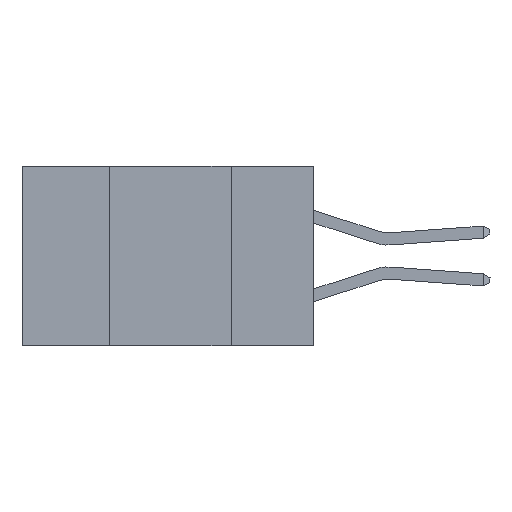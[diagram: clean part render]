
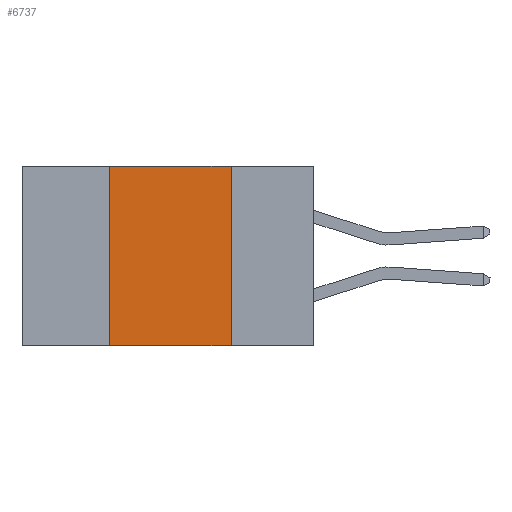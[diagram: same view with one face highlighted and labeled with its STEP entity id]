
A CAD part, left-side view. The second image highlights one B-rep face of the part: STEP entity #6737.
In plain terms, the highlighted planar face has unit normal (-1, 0, 0).
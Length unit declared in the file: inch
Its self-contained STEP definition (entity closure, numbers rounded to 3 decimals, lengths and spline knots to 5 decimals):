
#291 = EDGE_CURVE ( 'NONE', #8568, #8431, #4591, .T. ) ;
#351 = CARTESIAN_POINT ( 'NONE',  ( 0., 0.17, 0. ) ) ;
#398 = CARTESIAN_POINT ( 'NONE',  ( 0., 0.17, -0.37 ) ) ;
#444 = VERTEX_POINT ( 'NONE', #351 ) ;
#1081 = EDGE_LOOP ( 'NONE', ( #2497, #6283, #7245, #1813 ) ) ;
#1221 = FACE_OUTER_BOUND ( 'NONE', #1081, .T. ) ;
#1482 = LINE ( 'NONE', #3401, #9148 ) ;
#1788 = DIRECTION ( 'NONE',  ( 0., 0., -1. ) ) ;
#1813 = ORIENTED_EDGE ( 'NONE', *, *, #291, .T. ) ;
#2138 = DIRECTION ( 'NONE',  ( 0., -1., 0. ) ) ;
#2497 = ORIENTED_EDGE ( 'NONE', *, *, #6700, .F. ) ;
#3296 = EDGE_CURVE ( 'NONE', #9327, #444, #10441, .T. ) ;
#3401 = CARTESIAN_POINT ( 'NONE',  ( 0., 0.17, 0. ) ) ;
#3437 = CARTESIAN_POINT ( 'NONE',  ( 0., 0.6, 0. ) ) ;
#3501 = CARTESIAN_POINT ( 'NONE',  ( 0., 0.6, -0.37 ) ) ;
#3735 = CARTESIAN_POINT ( 'NONE',  ( 0., 0.6, 0. ) ) ;
#4591 = LINE ( 'NONE', #3501, #7602 ) ;
#4849 = LINE ( 'NONE', #8073, #6753 ) ;
#5057 = VECTOR ( 'NONE', #2138, 39.37008 ) ;
#5159 = DIRECTION ( 'NONE',  ( 0., 0., -1. ) ) ;
#6283 = ORIENTED_EDGE ( 'NONE', *, *, #3296, .F. ) ;
#6490 = CARTESIAN_POINT ( 'NONE',  ( 0., 0.42, -0.37 ) ) ;
#6700 = EDGE_CURVE ( 'NONE', #444, #8431, #1482, .T. ) ;
#6737 = ADVANCED_FACE ( 'NONE', ( #1221 ), #8248, .F. ) ;
#6753 = VECTOR ( 'NONE', #9820, 39.37008 ) ;
#7245 = ORIENTED_EDGE ( 'NONE', *, *, #7766, .F. ) ;
#7514 = AXIS2_PLACEMENT_3D ( 'NONE', #3437, #9862, #5159 ) ;
#7602 = VECTOR ( 'NONE', #9016, 39.37008 ) ;
#7675 = CARTESIAN_POINT ( 'NONE',  ( 0., 0.42, 0. ) ) ;
#7766 = EDGE_CURVE ( 'NONE', #8568, #9327, #4849, .T. ) ;
#8073 = CARTESIAN_POINT ( 'NONE',  ( 0., 0.42, 0. ) ) ;
#8248 = PLANE ( 'NONE',  #7514 ) ;
#8431 = VERTEX_POINT ( 'NONE', #398 ) ;
#8568 = VERTEX_POINT ( 'NONE', #6490 ) ;
#9016 = DIRECTION ( 'NONE',  ( 0., -1., 0. ) ) ;
#9148 = VECTOR ( 'NONE', #1788, 39.37008 ) ;
#9327 = VERTEX_POINT ( 'NONE', #7675 ) ;
#9820 = DIRECTION ( 'NONE',  ( 0., 0., 1. ) ) ;
#9862 = DIRECTION ( 'NONE',  ( 1., 0., 0. ) ) ;
#10441 = LINE ( 'NONE', #3735, #5057 ) ;
